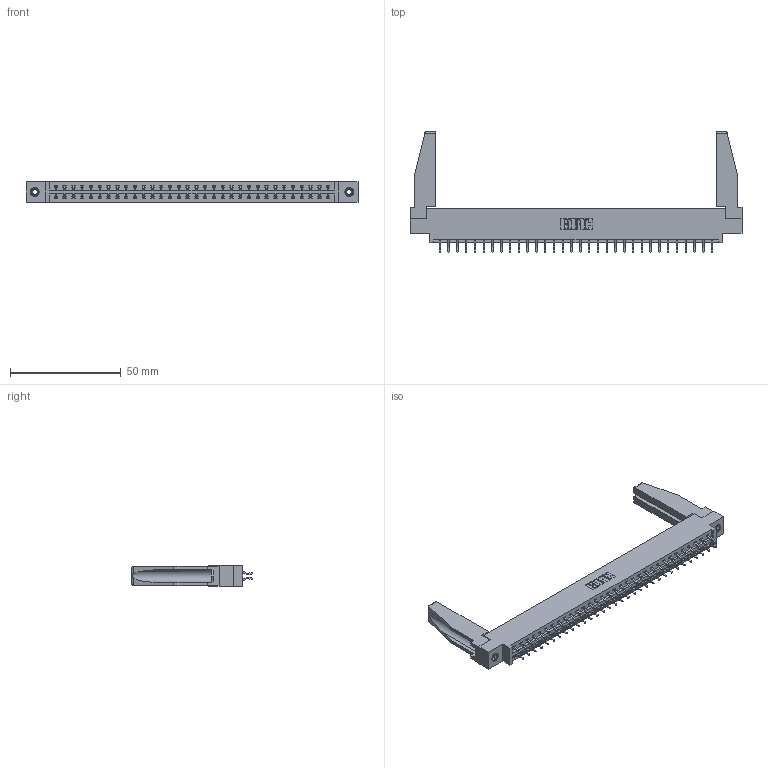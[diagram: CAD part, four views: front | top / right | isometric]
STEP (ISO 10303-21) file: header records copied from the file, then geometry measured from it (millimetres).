
FILE_DESCRIPTION (( 'STEP AP203' ), '1' );
FILE_NAME ('387-064-556-878.STEP', '2019-10-19T17:27:37', ( '' ), ( '' ), 'SwSTEP 2.0', 'SolidWorks 2016', '' );
FILE_SCHEMA (( 'CONFIG_CONTROL_DESIGN' ));
Length unit declared in the file: inch
Products named in the file (5): 387-064-556-878; 307-220-078; 345-250-001_345-250-001-102; 345-292-001_556 Tail; 337 Part_0.170 Offset - 0.156 Dia-TI
Assembly tree (69 placements, depth 2):
  387-064-556-878
    337 Part_0.170 Offset - 0.156 Dia-TI
    345-292-001_556 Tail  x64
    345-250-001_345-250-001-102  x2
    307-220-078  x2
Bounding box: 149.81 x 54.37 x 9.4 mm (x, y, z)
Volume: 19528.3 mm3; surface area: 21335.9 mm2
Topology: 69 solids, 69 shells, 4088 faces, 12109 edges, 7978 vertices
Faces by surface type: plane 2846, cylinder 1226, cone 12, torus 4
Entity records: 28896 total; most frequent: CARTESIAN_POINT 4892, ORIENTED_EDGE 4772, DIRECTION 4174, EDGE_CURVE 2386, LINE 2212, VECTOR 2212, VERTEX_POINT 1584, AXIS2_PLACEMENT_3D 981
